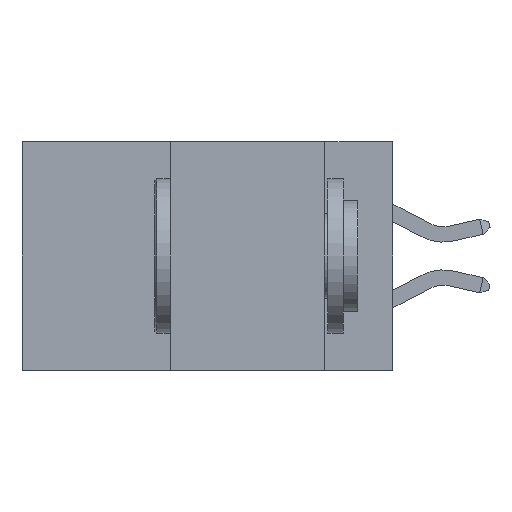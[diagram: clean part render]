
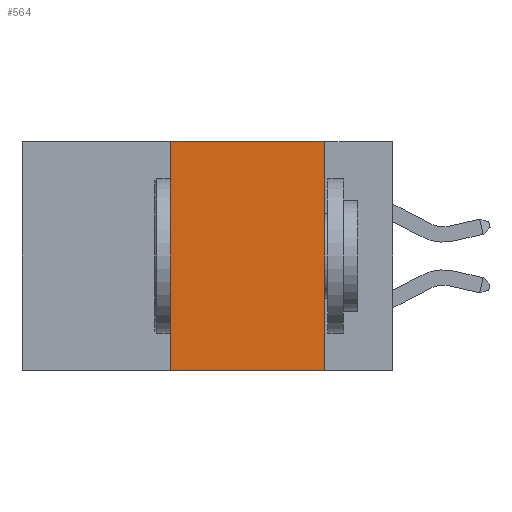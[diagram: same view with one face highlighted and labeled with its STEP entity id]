
A CAD part, left-side view. The second image highlights one B-rep face of the part: STEP entity #564.
In plain terms, the highlighted planar face has unit normal (-1, 0, 0).
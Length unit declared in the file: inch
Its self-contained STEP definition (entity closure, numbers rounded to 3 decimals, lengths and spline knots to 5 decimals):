
#447 = LINE ( 'NONE', #13648, #6537 ) ;
#564 = ADVANCED_FACE ( 'NONE', ( #12425 ), #8593, .F. ) ;
#852 = LINE ( 'NONE', #9144, #7257 ) ;
#1197 = ORIENTED_EDGE ( 'NONE', *, *, #13945, .T. ) ;
#1468 = VERTEX_POINT ( 'NONE', #14079 ) ;
#1604 = VERTEX_POINT ( 'NONE', #14136 ) ;
#2063 = VERTEX_POINT ( 'NONE', #14898 ) ;
#2705 = AXIS2_PLACEMENT_3D ( 'NONE', #4481, #4513, #7583 ) ;
#4132 = EDGE_LOOP ( 'NONE', ( #6663, #9648, #9490, #1197 ) ) ;
#4481 = CARTESIAN_POINT ( 'NONE',  ( 0., 0.6, 0. ) ) ;
#4513 = DIRECTION ( 'NONE',  ( 1., 0., 0. ) ) ;
#4673 = DIRECTION ( 'NONE',  ( 0., 0., 1. ) ) ;
#5596 = VERTEX_POINT ( 'NONE', #8492 ) ;
#6533 = LINE ( 'NONE', #10333, #6913 ) ;
#6537 = VECTOR ( 'NONE', #14771, 39.37008 ) ;
#6663 = ORIENTED_EDGE ( 'NONE', *, *, #13964, .F. ) ;
#6913 = VECTOR ( 'NONE', #4673, 39.37008 ) ;
#6954 = CARTESIAN_POINT ( 'NONE',  ( 0., 0.11, 0. ) ) ;
#7257 = VECTOR ( 'NONE', #10292, 39.37008 ) ;
#7583 = DIRECTION ( 'NONE',  ( 0., 0., -1. ) ) ;
#8492 = CARTESIAN_POINT ( 'NONE',  ( 0., 0.11, 0. ) ) ;
#8593 = PLANE ( 'NONE',  #2705 ) ;
#9144 = CARTESIAN_POINT ( 'NONE',  ( 0., 0.6, -0.37 ) ) ;
#9490 = ORIENTED_EDGE ( 'NONE', *, *, #13973, .F. ) ;
#9539 = VECTOR ( 'NONE', #11441, 39.37008 ) ;
#9648 = ORIENTED_EDGE ( 'NONE', *, *, #14412, .F. ) ;
#10292 = DIRECTION ( 'NONE',  ( 0., -1., 0. ) ) ;
#10333 = CARTESIAN_POINT ( 'NONE',  ( 0., 0.36, 0. ) ) ;
#11441 = DIRECTION ( 'NONE',  ( 0., 0., -1. ) ) ;
#12425 = FACE_OUTER_BOUND ( 'NONE', #4132, .T. ) ;
#13305 = LINE ( 'NONE', #6954, #9539 ) ;
#13648 = CARTESIAN_POINT ( 'NONE',  ( 0., 0.6, 0. ) ) ;
#13945 = EDGE_CURVE ( 'NONE', #1468, #2063, #852, .T. ) ;
#13964 = EDGE_CURVE ( 'NONE', #5596, #2063, #13305, .T. ) ;
#13973 = EDGE_CURVE ( 'NONE', #1468, #1604, #6533, .T. ) ;
#14079 = CARTESIAN_POINT ( 'NONE',  ( 0., 0.36, -0.37 ) ) ;
#14136 = CARTESIAN_POINT ( 'NONE',  ( 0., 0.36, 0. ) ) ;
#14412 = EDGE_CURVE ( 'NONE', #1604, #5596, #447, .T. ) ;
#14771 = DIRECTION ( 'NONE',  ( 0., -1., 0. ) ) ;
#14898 = CARTESIAN_POINT ( 'NONE',  ( 0., 0.11, -0.37 ) ) ;
